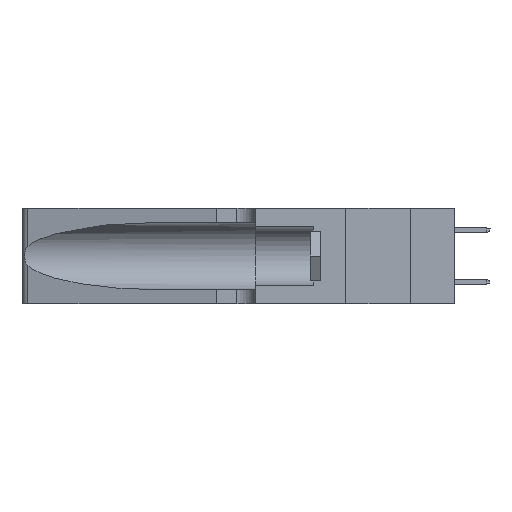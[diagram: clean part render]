
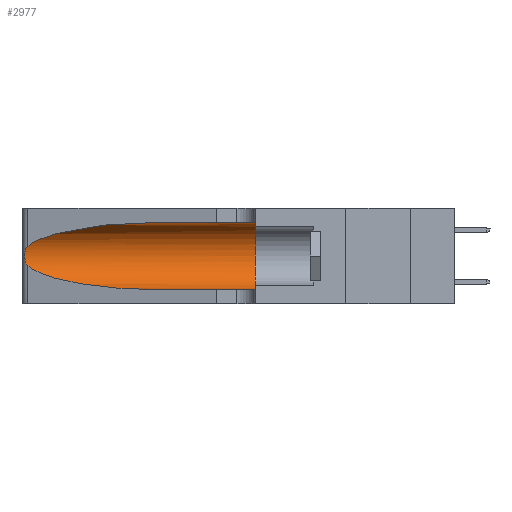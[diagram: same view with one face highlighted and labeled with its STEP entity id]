
A CAD part, left-side view. The second image highlights one B-rep face of the part: STEP entity #2977.
In plain terms, the highlighted cylindrical face has radius 3.308 mm (diameter 6.617 mm), a partial arc.
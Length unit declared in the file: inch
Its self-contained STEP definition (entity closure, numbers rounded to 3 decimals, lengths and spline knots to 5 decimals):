
#546 = VERTEX_POINT ( 'NONE', #16273 ) ;
#586 = DIRECTION ( 'NONE',  ( 0., -1., 0. ) ) ;
#816 = CARTESIAN_POINT ( 'NONE',  ( 0.1305, 1.61858, 0.31525 ) ) ;
#820 = AXIS2_PLACEMENT_3D ( 'NONE', #4270, #11324, #15313 ) ;
#1534 = CARTESIAN_POINT ( 'NONE',  ( 0.2373, 1.15595, 0.08982 ) ) ;
#1938 = CARTESIAN_POINT ( 'NONE',  ( 0.1305, 0.72297, 0.31525 ) ) ;
#2113 = CYLINDRICAL_SURFACE ( 'NONE', #820, 0.13025 ) ;
#2382 = LINE ( 'NONE', #14803, #5794 ) ;
#2392 = ORIENTED_EDGE ( 'NONE', *, *, #6184, .T. ) ;
#2977 = ADVANCED_FACE ( 'NONE', ( #8145 ), #2113, .F. ) ;
#3265 = CARTESIAN_POINT ( 'NONE',  ( 0.25487, 1.22718, 0.22369 ) ) ;
#3374 = CARTESIAN_POINT ( 'NONE',  ( 0.26075, 1.23896, 0.19203 ) ) ;
#4041 = EDGE_CURVE ( 'NONE', #16120, #10153, #22529, .T. ) ;
#4270 = CARTESIAN_POINT ( 'NONE',  ( 0.1305, 1.61858, 0.185 ) ) ;
#4830 = CARTESIAN_POINT ( 'NONE',  ( 0.1305, 0.35, 0.05475 ) ) ;
#4867 = CARTESIAN_POINT ( 'NONE',  ( 0.25787, 1.23484, 0.2124 ) ) ;
#4990 = CARTESIAN_POINT ( 'NONE',  ( 0.2373, 1.15595, 0.28018 ) ) ;
#5215 = CARTESIAN_POINT ( 'NONE',  ( 0.26017, 1.23833, 0.17102 ) ) ;
#5478 = VERTEX_POINT ( 'NONE', #11900 ) ;
#5794 = VECTOR ( 'NONE', #586, 39.37008 ) ;
#5819 = CARTESIAN_POINT ( 'NONE',  ( 0.25487, 1.22718, 0.14631 ) ) ;
#6100 = ORIENTED_EDGE ( 'NONE', *, *, #12317, .T. ) ;
#6184 = EDGE_CURVE ( 'NONE', #18197, #20493, #2382, .T. ) ;
#6423 = CARTESIAN_POINT ( 'NONE',  ( 0.1305, 0.72297, 0.05475 ) ) ;
#6820 = CARTESIAN_POINT ( 'NONE',  ( 0.18966, 0.96281, 0.05475 ) ) ;
#6900 = CARTESIAN_POINT ( 'NONE',  ( 0.26075, 1.23896, 0.178 ) ) ;
#7828 = ORIENTED_EDGE ( 'NONE', *, *, #21456, .F. ) ;
#8145 = FACE_OUTER_BOUND ( 'NONE', #21558, .T. ) ;
#8536 = CARTESIAN_POINT ( 'NONE',  ( 0.25639, 1.23184, 0.21858 ) ) ;
#8604 = EDGE_CURVE ( 'NONE', #10153, #18197, #10111, .T. ) ;
#10111 =( BOUNDED_CURVE ( )  B_SPLINE_CURVE ( 3, ( #17455, #1534, #6820, #13954 ),
 .UNSPECIFIED., .F., .F. ) 
 B_SPLINE_CURVE_WITH_KNOTS ( ( 4, 4 ),
 ( 3.44316, 4.71239 ),
 .UNSPECIFIED. ) 
 CURVE ( )  GEOMETRIC_REPRESENTATION_ITEM ( )  RATIONAL_B_SPLINE_CURVE ( ( 1., 0.87, 0.87, 1. ) ) 
 REPRESENTATION_ITEM ( '' )  );
#10153 = VERTEX_POINT ( 'NONE', #5819 ) ;
#11324 = DIRECTION ( 'NONE',  ( 0., -1., 0. ) ) ;
#11327 = ORIENTED_EDGE ( 'NONE', *, *, #4041, .T. ) ;
#11900 = CARTESIAN_POINT ( 'NONE',  ( 0.1305, 0.72297, 0.31525 ) ) ;
#12267 = CARTESIAN_POINT ( 'NONE',  ( 0.25854, 1.2359, 0.20912 ) ) ;
#12317 = EDGE_CURVE ( 'NONE', #5478, #16120, #14173, .T. ) ;
#12390 = CARTESIAN_POINT ( 'NONE',  ( 0.25555, 1.22994, 0.2215 ) ) ;
#12410 = EDGE_CURVE ( 'NONE', #546, #20493, #16710, .T. ) ;
#12721 = ORIENTED_EDGE ( 'NONE', *, *, #12410, .F. ) ;
#13954 = CARTESIAN_POINT ( 'NONE',  ( 0.1305, 0.72297, 0.05475 ) ) ;
#14154 = CARTESIAN_POINT ( 'NONE',  ( 0.25487, 1.22718, 0.14631 ) ) ;
#14173 =( BOUNDED_CURVE ( )  B_SPLINE_CURVE ( 3, ( #1938, #14253, #4990, #20899 ),
 .UNSPECIFIED., .F., .F. ) 
 B_SPLINE_CURVE_WITH_KNOTS ( ( 4, 4 ),
 ( 1.5708, 2.84003 ),
 .UNSPECIFIED. ) 
 CURVE ( )  GEOMETRIC_REPRESENTATION_ITEM ( )  RATIONAL_B_SPLINE_CURVE ( ( 1., 0.87, 0.87, 1. ) ) 
 REPRESENTATION_ITEM ( '' )  );
#14253 = CARTESIAN_POINT ( 'NONE',  ( 0.18966, 0.96281, 0.31525 ) ) ;
#14803 = CARTESIAN_POINT ( 'NONE',  ( 0.1305, 1.61858, 0.05475 ) ) ;
#15313 = DIRECTION ( 'NONE',  ( 0., 0., -1. ) ) ;
#15360 = DIRECTION ( 'NONE',  ( 0., -1., 0. ) ) ;
#15688 = CARTESIAN_POINT ( 'NONE',  ( 0.26018, 1.23835, 0.19895 ) ) ;
#16120 = VERTEX_POINT ( 'NONE', #16513 ) ;
#16273 = CARTESIAN_POINT ( 'NONE',  ( 0.1305, 0.35, 0.31525 ) ) ;
#16431 = ORIENTED_EDGE ( 'NONE', *, *, #8604, .T. ) ;
#16513 = CARTESIAN_POINT ( 'NONE',  ( 0.25487, 1.22718, 0.22369 ) ) ;
#16575 = DIRECTION ( 'NONE',  ( 0., 1., 0. ) ) ;
#16710 = CIRCLE ( 'NONE', #19678, 0.13025 ) ;
#17455 = CARTESIAN_POINT ( 'NONE',  ( 0.25487, 1.22718, 0.14631 ) ) ;
#17653 = CARTESIAN_POINT ( 'NONE',  ( 0.25555, 1.22993, 0.14849 ) ) ;
#18088 = CARTESIAN_POINT ( 'NONE',  ( 0.1305, 0.35, 0.185 ) ) ;
#18197 = VERTEX_POINT ( 'NONE', #6423 ) ;
#19491 = CARTESIAN_POINT ( 'NONE',  ( 0.25639, 1.23186, 0.15144 ) ) ;
#19678 = AXIS2_PLACEMENT_3D ( 'NONE', #18088, #16575, #21802 ) ;
#20318 = VECTOR ( 'NONE', #15360, 39.37008 ) ;
#20493 = VERTEX_POINT ( 'NONE', #4830 ) ;
#20576 = LINE ( 'NONE', #816, #20318 ) ;
#20899 = CARTESIAN_POINT ( 'NONE',  ( 0.25487, 1.22718, 0.22369 ) ) ;
#21456 = EDGE_CURVE ( 'NONE', #5478, #546, #20576, .T. ) ;
#21558 = EDGE_LOOP ( 'NONE', ( #6100, #11327, #16431, #2392, #12721, #7828 ) ) ;
#21802 = DIRECTION ( 'NONE',  ( 0., 0., 1. ) ) ;
#22529 = B_SPLINE_CURVE_WITH_KNOTS ( 'NONE', 3,
 ( #3265, #12390, #8536, #4867, #12267, #15688, #3374, #6900, #5215, #22748, #22970, #19491, #17653, #14154 ),
 .UNSPECIFIED., .F., .F.,
 ( 4, 2, 2, 2, 2, 2, 4 ),
 ( 0., 0.00027, 0.00053, 0.00107, 0.0016, 0.00187, 0.00214 ),
 .UNSPECIFIED. ) ;
#22748 = CARTESIAN_POINT ( 'NONE',  ( 0.25856, 1.23593, 0.16098 ) ) ;
#22970 = CARTESIAN_POINT ( 'NONE',  ( 0.25789, 1.23486, 0.15765 ) ) ;
